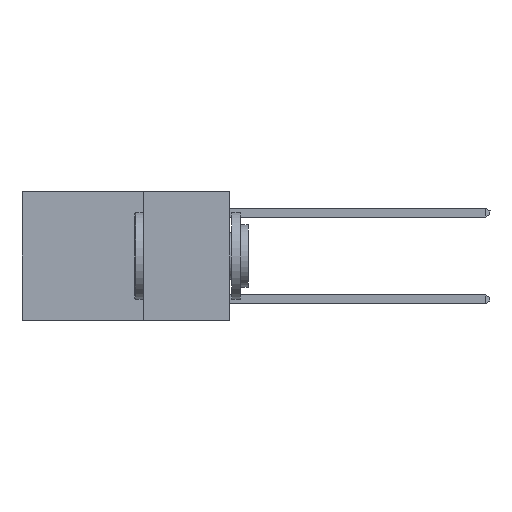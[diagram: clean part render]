
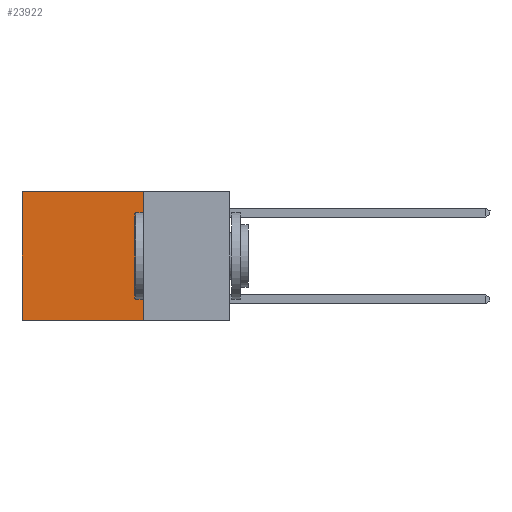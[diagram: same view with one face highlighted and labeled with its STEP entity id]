
A CAD part, left-side view. The second image highlights one B-rep face of the part: STEP entity #23922.
In plain terms, the highlighted planar face has unit normal (-1, 0, 0).
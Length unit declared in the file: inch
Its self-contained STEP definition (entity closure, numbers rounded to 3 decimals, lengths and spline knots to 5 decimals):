
#1281 = CARTESIAN_POINT ( 'NONE',  ( 0.2625, 0.6, 0. ) ) ;
#1481 = DIRECTION ( 'NONE',  ( 0., 0., -1. ) ) ;
#1744 = VECTOR ( 'NONE', #10919, 39.37008 ) ;
#2078 = VERTEX_POINT ( 'NONE', #7998 ) ;
#2298 = EDGE_CURVE ( 'NONE', #2078, #12244, #11302, .T. ) ;
#2429 = DIRECTION ( 'NONE',  ( 0., 1., 0. ) ) ;
#2754 = EDGE_CURVE ( 'NONE', #2078, #14179, #23081, .T. ) ;
#3588 = CARTESIAN_POINT ( 'NONE',  ( 0.2625, 0.25, 0. ) ) ;
#3663 = LINE ( 'NONE', #1281, #1744 ) ;
#5328 = DIRECTION ( 'NONE',  ( 1., 0., 0. ) ) ;
#7342 = ORIENTED_EDGE ( 'NONE', *, *, #27541, .F. ) ;
#7998 = CARTESIAN_POINT ( 'NONE',  ( 0.2625, 0.25, 0. ) ) ;
#10462 = CARTESIAN_POINT ( 'NONE',  ( 0.2625, 0.6, 0. ) ) ;
#10919 = DIRECTION ( 'NONE',  ( 0., 0., -1. ) ) ;
#11302 = LINE ( 'NONE', #30522, #11941 ) ;
#11941 = VECTOR ( 'NONE', #18382, 39.37008 ) ;
#12244 = VERTEX_POINT ( 'NONE', #10462 ) ;
#12250 = AXIS2_PLACEMENT_3D ( 'NONE', #3588, #5328, #24850 ) ;
#13295 = ORIENTED_EDGE ( 'NONE', *, *, #2298, .T. ) ;
#13604 = VECTOR ( 'NONE', #1481, 39.37008 ) ;
#14179 = VERTEX_POINT ( 'NONE', #17992 ) ;
#17402 = VERTEX_POINT ( 'NONE', #29172 ) ;
#17992 = CARTESIAN_POINT ( 'NONE',  ( 0.2625, 0.25, -0.37 ) ) ;
#18088 = PLANE ( 'NONE',  #12250 ) ;
#18382 = DIRECTION ( 'NONE',  ( 0., 1., 0. ) ) ;
#18919 = EDGE_CURVE ( 'NONE', #12244, #17402, #3663, .T. ) ;
#19599 = LINE ( 'NONE', #24012, #24915 ) ;
#23081 = LINE ( 'NONE', #25434, #13604 ) ;
#23922 = ADVANCED_FACE ( 'NONE', ( #25169 ), #18088, .F. ) ;
#24012 = CARTESIAN_POINT ( 'NONE',  ( 0.2625, 0.25, -0.37 ) ) ;
#24850 = DIRECTION ( 'NONE',  ( 0., 0., -1. ) ) ;
#24915 = VECTOR ( 'NONE', #2429, 39.37008 ) ;
#25169 = FACE_OUTER_BOUND ( 'NONE', #26322, .T. ) ;
#25300 = ORIENTED_EDGE ( 'NONE', *, *, #18919, .T. ) ;
#25434 = CARTESIAN_POINT ( 'NONE',  ( 0.2625, 0.25, 0. ) ) ;
#26322 = EDGE_LOOP ( 'NONE', ( #25300, #7342, #30619, #13295 ) ) ;
#27541 = EDGE_CURVE ( 'NONE', #14179, #17402, #19599, .T. ) ;
#29172 = CARTESIAN_POINT ( 'NONE',  ( 0.2625, 0.6, -0.37 ) ) ;
#30522 = CARTESIAN_POINT ( 'NONE',  ( 0.2625, 0.25, 0. ) ) ;
#30619 = ORIENTED_EDGE ( 'NONE', *, *, #2754, .F. ) ;
